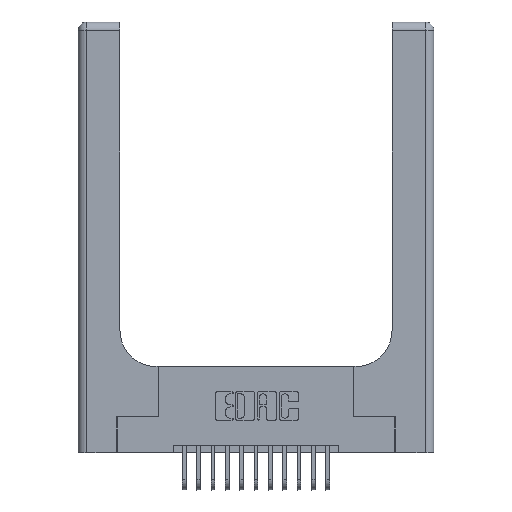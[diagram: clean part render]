
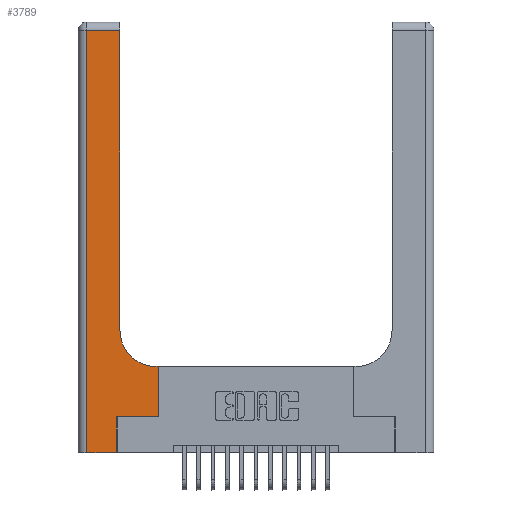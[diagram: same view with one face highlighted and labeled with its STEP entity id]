
A CAD part, top view. The second image highlights one B-rep face of the part: STEP entity #3789.
In plain terms, the highlighted planar face has unit normal (0, 0, 1).
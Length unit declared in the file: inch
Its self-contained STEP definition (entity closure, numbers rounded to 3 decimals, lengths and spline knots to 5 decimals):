
#74 = LINE ( 'NONE', #16712, #9148 ) ;
#135 = DIRECTION ( 'NONE',  ( 0., 1., 0. ) ) ;
#250 = EDGE_CURVE ( 'NONE', #3405, #12191, #4841, .T. ) ;
#289 = VERTEX_POINT ( 'NONE', #16582 ) ;
#337 = CARTESIAN_POINT ( 'NONE',  ( 0.2915, 3., 0.37 ) ) ;
#473 = LINE ( 'NONE', #10821, #19673 ) ;
#984 = DIRECTION ( 'NONE',  ( 0., 0., -1. ) ) ;
#1079 = ORIENTED_EDGE ( 'NONE', *, *, #250, .T. ) ;
#1809 = ORIENTED_EDGE ( 'NONE', *, *, #17019, .T. ) ;
#1815 = AXIS2_PLACEMENT_3D ( 'NONE', #5981, #12044, #4447 ) ;
#2094 = DIRECTION ( 'NONE',  ( -1., 0., 0. ) ) ;
#2252 = LINE ( 'NONE', #18322, #11304 ) ;
#2582 = PLANE ( 'NONE',  #15225 ) ;
#2588 = EDGE_CURVE ( 'NONE', #7632, #3405, #473, .T. ) ;
#2983 = EDGE_CURVE ( 'NONE', #10436, #289, #10929, .T. ) ;
#3355 = ORIENTED_EDGE ( 'NONE', *, *, #13908, .T. ) ;
#3366 = DIRECTION ( 'NONE',  ( 0., 1., 0. ) ) ;
#3405 = VERTEX_POINT ( 'NONE', #19535 ) ;
#3504 = VECTOR ( 'NONE', #2094, 39.37008 ) ;
#3789 = ADVANCED_FACE ( 'NONE', ( #3998 ), #2582, .F. ) ;
#3985 = VECTOR ( 'NONE', #10146, 39.37008 ) ;
#3986 = VERTEX_POINT ( 'NONE', #5470 ) ;
#3998 = FACE_OUTER_BOUND ( 'NONE', #15867, .T. ) ;
#4447 = DIRECTION ( 'NONE',  ( 1., 0., 0. ) ) ;
#4567 = CARTESIAN_POINT ( 'NONE',  ( 0.5585, 0.25, 0.37 ) ) ;
#4841 = CIRCLE ( 'NONE', #1815, 0.25 ) ;
#5470 = CARTESIAN_POINT ( 'NONE',  ( 0.269, 0., 0.37 ) ) ;
#5981 = CARTESIAN_POINT ( 'NONE',  ( 0.5415, 0.85, 0.37 ) ) ;
#6179 = CARTESIAN_POINT ( 'NONE',  ( 0.06, 3., 0.37 ) ) ;
#6253 = DIRECTION ( 'NONE',  ( 0., -1., 0. ) ) ;
#6647 = CARTESIAN_POINT ( 'NONE',  ( 0.2915, 2.94, 0.37 ) ) ;
#6833 = LINE ( 'NONE', #337, #14676 ) ;
#6970 = ORIENTED_EDGE ( 'NONE', *, *, #2588, .T. ) ;
#7108 = CARTESIAN_POINT ( 'NONE',  ( 0.5585, 0.25, 0.37 ) ) ;
#7632 = VERTEX_POINT ( 'NONE', #8969 ) ;
#8183 = ORIENTED_EDGE ( 'NONE', *, *, #17339, .T. ) ;
#8516 = LINE ( 'NONE', #19157, #3985 ) ;
#8969 = CARTESIAN_POINT ( 'NONE',  ( 0.5585, 0.6, 0.37 ) ) ;
#9148 = VECTOR ( 'NONE', #15281, 39.37008 ) ;
#9191 = CARTESIAN_POINT ( 'NONE',  ( 0.269, 0.25, 0.37 ) ) ;
#10146 = DIRECTION ( 'NONE',  ( 1., 0., 0. ) ) ;
#10436 = VERTEX_POINT ( 'NONE', #6647 ) ;
#10772 = VERTEX_POINT ( 'NONE', #7108 ) ;
#10821 = CARTESIAN_POINT ( 'NONE',  ( 0.2915, 0.6, 0.37 ) ) ;
#10929 = LINE ( 'NONE', #13180, #3504 ) ;
#11304 = VECTOR ( 'NONE', #135, 39.37008 ) ;
#12044 = DIRECTION ( 'NONE',  ( 0., 0., -1. ) ) ;
#12191 = VERTEX_POINT ( 'NONE', #19654 ) ;
#12397 = DIRECTION ( 'NONE',  ( 0., 1., 0. ) ) ;
#13180 = CARTESIAN_POINT ( 'NONE',  ( 0., 2.94, 0.37 ) ) ;
#13265 = VECTOR ( 'NONE', #6253, 39.37008 ) ;
#13732 = LINE ( 'NONE', #6179, #13265 ) ;
#13908 = EDGE_CURVE ( 'NONE', #12191, #10436, #6833, .T. ) ;
#14094 = EDGE_CURVE ( 'NONE', #289, #14872, #13732, .T. ) ;
#14436 = EDGE_CURVE ( 'NONE', #16298, #10772, #8516, .T. ) ;
#14676 = VECTOR ( 'NONE', #12397, 39.37008 ) ;
#14872 = VERTEX_POINT ( 'NONE', #14905 ) ;
#14905 = CARTESIAN_POINT ( 'NONE',  ( 0.06, 0., 0.37 ) ) ;
#15197 = ORIENTED_EDGE ( 'NONE', *, *, #14094, .T. ) ;
#15225 = AXIS2_PLACEMENT_3D ( 'NONE', #19267, #984, #16373 ) ;
#15281 = DIRECTION ( 'NONE',  ( 1., 0., 0. ) ) ;
#15437 = ORIENTED_EDGE ( 'NONE', *, *, #2983, .T. ) ;
#15562 = DIRECTION ( 'NONE',  ( -1., 0., 0. ) ) ;
#15867 = EDGE_LOOP ( 'NONE', ( #3355, #15437, #15197, #8183, #1809, #18548, #16237, #6970, #1079 ) ) ;
#16237 = ORIENTED_EDGE ( 'NONE', *, *, #18109, .T. ) ;
#16298 = VERTEX_POINT ( 'NONE', #9191 ) ;
#16373 = DIRECTION ( 'NONE',  ( -1., 0., 0. ) ) ;
#16582 = CARTESIAN_POINT ( 'NONE',  ( 0.06, 2.94, 0.37 ) ) ;
#16659 = LINE ( 'NONE', #4567, #19032 ) ;
#16712 = CARTESIAN_POINT ( 'NONE',  ( 0., 0., 0.37 ) ) ;
#17019 = EDGE_CURVE ( 'NONE', #3986, #16298, #2252, .T. ) ;
#17339 = EDGE_CURVE ( 'NONE', #14872, #3986, #74, .T. ) ;
#18109 = EDGE_CURVE ( 'NONE', #10772, #7632, #16659, .T. ) ;
#18322 = CARTESIAN_POINT ( 'NONE',  ( 0.269, 0., 0.37 ) ) ;
#18548 = ORIENTED_EDGE ( 'NONE', *, *, #14436, .T. ) ;
#19032 = VECTOR ( 'NONE', #3366, 39.37008 ) ;
#19157 = CARTESIAN_POINT ( 'NONE',  ( 0.269, 0.25, 0.37 ) ) ;
#19267 = CARTESIAN_POINT ( 'NONE',  ( 0., 3., 0.37 ) ) ;
#19535 = CARTESIAN_POINT ( 'NONE',  ( 0.5415, 0.6, 0.37 ) ) ;
#19654 = CARTESIAN_POINT ( 'NONE',  ( 0.2915, 0.85, 0.37 ) ) ;
#19673 = VECTOR ( 'NONE', #15562, 39.37008 ) ;
